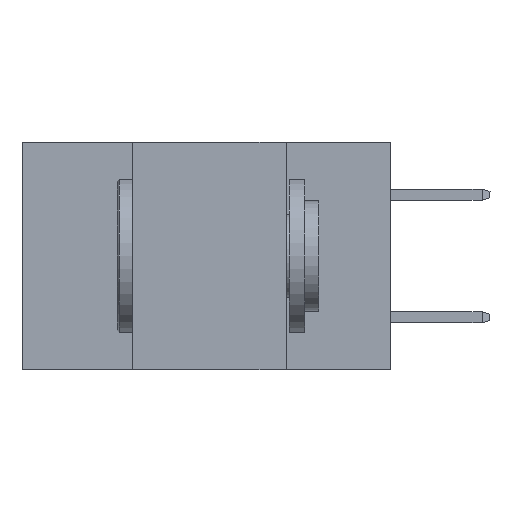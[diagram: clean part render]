
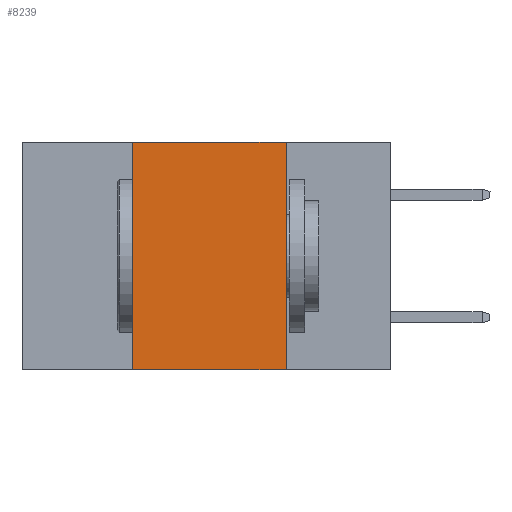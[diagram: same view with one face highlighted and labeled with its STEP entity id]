
A CAD part, left-side view. The second image highlights one B-rep face of the part: STEP entity #8239.
In plain terms, the highlighted planar face has unit normal (-1, 0, 0).
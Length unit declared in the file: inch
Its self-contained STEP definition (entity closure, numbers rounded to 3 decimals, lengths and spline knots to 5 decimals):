
#241 = LINE ( 'NONE', #10492, #3210 ) ;
#760 = EDGE_LOOP ( 'NONE', ( #1733, #5433, #2518, #12225 ) ) ;
#1051 = DIRECTION ( 'NONE',  ( 1., 0., 0. ) ) ;
#1489 = VECTOR ( 'NONE', #14315, 39.37008 ) ;
#1733 = ORIENTED_EDGE ( 'NONE', *, *, #3372, .F. ) ;
#1956 = VERTEX_POINT ( 'NONE', #14629 ) ;
#2518 = ORIENTED_EDGE ( 'NONE', *, *, #3472, .F. ) ;
#2742 = AXIS2_PLACEMENT_3D ( 'NONE', #14281, #1051, #9653 ) ;
#3210 = VECTOR ( 'NONE', #9264, 39.37008 ) ;
#3372 = EDGE_CURVE ( 'NONE', #6055, #1956, #3844, .T. ) ;
#3472 = EDGE_CURVE ( 'NONE', #12246, #14110, #8804, .T. ) ;
#3844 = LINE ( 'NONE', #11217, #7132 ) ;
#3996 = EDGE_CURVE ( 'NONE', #12246, #1956, #4805, .T. ) ;
#4805 = LINE ( 'NONE', #14414, #1489 ) ;
#5373 = EDGE_CURVE ( 'NONE', #14110, #6055, #241, .T. ) ;
#5433 = ORIENTED_EDGE ( 'NONE', *, *, #5373, .F. ) ;
#5899 = CARTESIAN_POINT ( 'NONE',  ( 0., 0.42, 0. ) ) ;
#6055 = VERTEX_POINT ( 'NONE', #12865 ) ;
#7132 = VECTOR ( 'NONE', #9624, 39.37008 ) ;
#7612 = CARTESIAN_POINT ( 'NONE',  ( 0., 0.42, 0. ) ) ;
#8024 = DIRECTION ( 'NONE',  ( 0., 0., 1. ) ) ;
#8239 = ADVANCED_FACE ( 'NONE', ( #12868 ), #13151, .F. ) ;
#8804 = LINE ( 'NONE', #5899, #12369 ) ;
#9264 = DIRECTION ( 'NONE',  ( 0., -1., 0. ) ) ;
#9624 = DIRECTION ( 'NONE',  ( 0., 0., -1. ) ) ;
#9653 = DIRECTION ( 'NONE',  ( 0., 0., -1. ) ) ;
#10492 = CARTESIAN_POINT ( 'NONE',  ( 0., 0.6, 0. ) ) ;
#11217 = CARTESIAN_POINT ( 'NONE',  ( 0., 0.17, 0. ) ) ;
#11959 = CARTESIAN_POINT ( 'NONE',  ( 0., 0.42, -0.37 ) ) ;
#12225 = ORIENTED_EDGE ( 'NONE', *, *, #3996, .T. ) ;
#12246 = VERTEX_POINT ( 'NONE', #11959 ) ;
#12369 = VECTOR ( 'NONE', #8024, 39.37008 ) ;
#12865 = CARTESIAN_POINT ( 'NONE',  ( 0., 0.17, 0. ) ) ;
#12868 = FACE_OUTER_BOUND ( 'NONE', #760, .T. ) ;
#13151 = PLANE ( 'NONE',  #2742 ) ;
#14110 = VERTEX_POINT ( 'NONE', #7612 ) ;
#14281 = CARTESIAN_POINT ( 'NONE',  ( 0., 0.6, 0. ) ) ;
#14315 = DIRECTION ( 'NONE',  ( 0., -1., 0. ) ) ;
#14414 = CARTESIAN_POINT ( 'NONE',  ( 0., 0.6, -0.37 ) ) ;
#14629 = CARTESIAN_POINT ( 'NONE',  ( 0., 0.17, -0.37 ) ) ;
